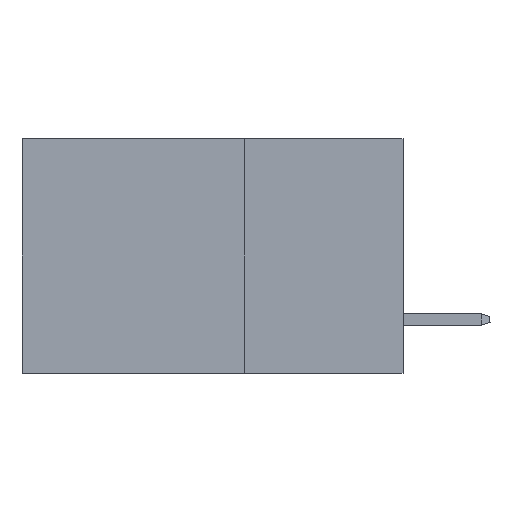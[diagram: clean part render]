
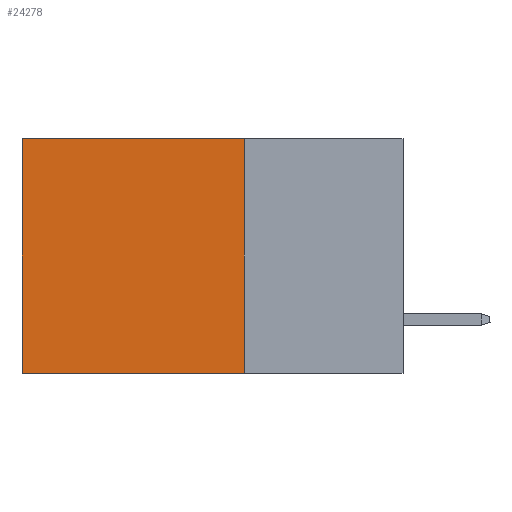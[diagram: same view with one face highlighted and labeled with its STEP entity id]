
A CAD part, left-side view. The second image highlights one B-rep face of the part: STEP entity #24278.
In plain terms, the highlighted planar face has unit normal (-1, 0, 0).
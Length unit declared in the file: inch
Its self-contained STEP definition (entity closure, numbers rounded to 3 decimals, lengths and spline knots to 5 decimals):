
#282 = CARTESIAN_POINT ( 'NONE',  ( 0.2875, 0.6, -0.37 ) ) ;
#315 = EDGE_LOOP ( 'NONE', ( #10672, #21325, #27633, #28204 ) ) ;
#573 = AXIS2_PLACEMENT_3D ( 'NONE', #21409, #5997, #14808 ) ;
#3419 = LINE ( 'NONE', #5626, #22258 ) ;
#5335 = DIRECTION ( 'NONE',  ( 0., 1., 0. ) ) ;
#5626 = CARTESIAN_POINT ( 'NONE',  ( 0.2875, 0.6, 0. ) ) ;
#5997 = DIRECTION ( 'NONE',  ( 1., 0., 0. ) ) ;
#7214 = LINE ( 'NONE', #16032, #12840 ) ;
#8100 = FACE_OUTER_BOUND ( 'NONE', #315, .T. ) ;
#9066 = VERTEX_POINT ( 'NONE', #12199 ) ;
#9845 = EDGE_CURVE ( 'NONE', #9066, #27806, #18639, .T. ) ;
#9937 = DIRECTION ( 'NONE',  ( 0., 0., -1. ) ) ;
#10550 = VERTEX_POINT ( 'NONE', #282 ) ;
#10672 = ORIENTED_EDGE ( 'NONE', *, *, #15812, .T. ) ;
#11511 = EDGE_CURVE ( 'NONE', #9066, #14455, #7214, .T. ) ;
#11713 = VECTOR ( 'NONE', #26031, 39.37008 ) ;
#12199 = CARTESIAN_POINT ( 'NONE',  ( 0.2875, 0.25, 0. ) ) ;
#12588 = PLANE ( 'NONE',  #573 ) ;
#12840 = VECTOR ( 'NONE', #9937, 39.37008 ) ;
#14157 = CARTESIAN_POINT ( 'NONE',  ( 0.2875, 0.25, 0. ) ) ;
#14455 = VERTEX_POINT ( 'NONE', #26611 ) ;
#14808 = DIRECTION ( 'NONE',  ( 0., 0., -1. ) ) ;
#15039 = LINE ( 'NONE', #19675, #11713 ) ;
#15812 = EDGE_CURVE ( 'NONE', #27806, #10550, #3419, .T. ) ;
#16032 = CARTESIAN_POINT ( 'NONE',  ( 0.2875, 0.25, 0. ) ) ;
#18639 = LINE ( 'NONE', #14157, #28049 ) ;
#19675 = CARTESIAN_POINT ( 'NONE',  ( 0.2875, 0.25, -0.37 ) ) ;
#21239 = DIRECTION ( 'NONE',  ( 0., 0., -1. ) ) ;
#21325 = ORIENTED_EDGE ( 'NONE', *, *, #26778, .F. ) ;
#21409 = CARTESIAN_POINT ( 'NONE',  ( 0.2875, 0.25, 0. ) ) ;
#22258 = VECTOR ( 'NONE', #21239, 39.37008 ) ;
#24278 = ADVANCED_FACE ( 'NONE', ( #8100 ), #12588, .F. ) ;
#26031 = DIRECTION ( 'NONE',  ( 0., 1., 0. ) ) ;
#26611 = CARTESIAN_POINT ( 'NONE',  ( 0.2875, 0.25, -0.37 ) ) ;
#26778 = EDGE_CURVE ( 'NONE', #14455, #10550, #15039, .T. ) ;
#26838 = CARTESIAN_POINT ( 'NONE',  ( 0.2875, 0.6, 0. ) ) ;
#27633 = ORIENTED_EDGE ( 'NONE', *, *, #11511, .F. ) ;
#27806 = VERTEX_POINT ( 'NONE', #26838 ) ;
#28049 = VECTOR ( 'NONE', #5335, 39.37008 ) ;
#28204 = ORIENTED_EDGE ( 'NONE', *, *, #9845, .T. ) ;
